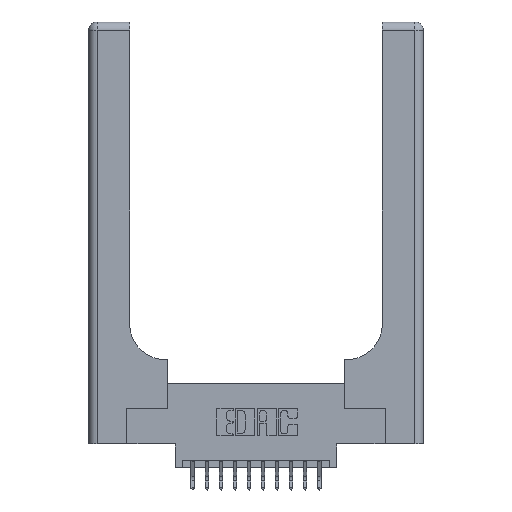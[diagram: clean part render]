
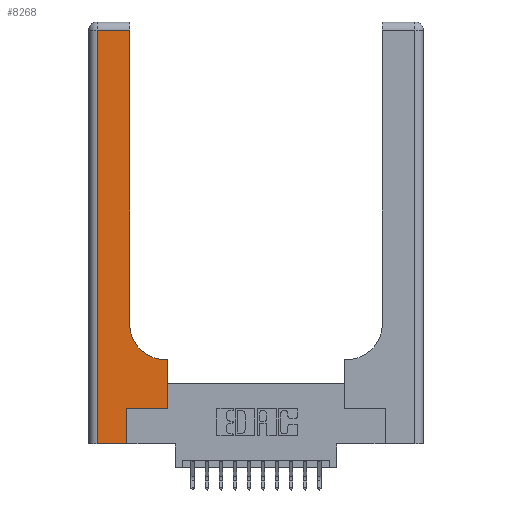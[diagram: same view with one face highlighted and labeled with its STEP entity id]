
A CAD part, top view. The second image highlights one B-rep face of the part: STEP entity #8268.
In plain terms, the highlighted planar face has unit normal (0, 0, 1).
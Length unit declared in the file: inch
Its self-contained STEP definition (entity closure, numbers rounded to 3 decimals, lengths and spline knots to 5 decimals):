
#43 = EDGE_CURVE ( 'NONE', #12131, #6065, #13467, .T. ) ;
#388 = CARTESIAN_POINT ( 'NONE',  ( 0.2915, 0.6, 0.37 ) ) ;
#536 = VECTOR ( 'NONE', #3226, 39.37008 ) ;
#683 = EDGE_CURVE ( 'NONE', #10627, #5318, #9512, .T. ) ;
#843 = CARTESIAN_POINT ( 'NONE',  ( 0., 0., 0.37 ) ) ;
#898 = ORIENTED_EDGE ( 'NONE', *, *, #2068, .T. ) ;
#954 = AXIS2_PLACEMENT_3D ( 'NONE', #13021, #5045, #14367 ) ;
#1008 = LINE ( 'NONE', #12621, #536 ) ;
#1689 = CARTESIAN_POINT ( 'NONE',  ( 0.06, 2.94, 0.37 ) ) ;
#2019 = CARTESIAN_POINT ( 'NONE',  ( 0.269, 0.25, 0.37 ) ) ;
#2068 = EDGE_CURVE ( 'NONE', #7461, #10627, #8013, .T. ) ;
#2261 = VECTOR ( 'NONE', #15564, 39.37008 ) ;
#3097 = DIRECTION ( 'NONE',  ( -1., 0., 0. ) ) ;
#3226 = DIRECTION ( 'NONE',  ( 0., 1., 0. ) ) ;
#3343 = DIRECTION ( 'NONE',  ( 0., -1., 0. ) ) ;
#4192 = EDGE_CURVE ( 'NONE', #5415, #10243, #4500, .T. ) ;
#4274 = ORIENTED_EDGE ( 'NONE', *, *, #10267, .T. ) ;
#4484 = CARTESIAN_POINT ( 'NONE',  ( 0., 2.94, 0.37 ) ) ;
#4500 = LINE ( 'NONE', #4484, #4947 ) ;
#4870 = DIRECTION ( 'NONE',  ( 1., 0., 0. ) ) ;
#4947 = VECTOR ( 'NONE', #3097, 39.37008 ) ;
#5045 = DIRECTION ( 'NONE',  ( 0., 0., -1. ) ) ;
#5318 = VERTEX_POINT ( 'NONE', #13586 ) ;
#5415 = VERTEX_POINT ( 'NONE', #11178 ) ;
#6065 = VERTEX_POINT ( 'NONE', #7530 ) ;
#6084 = CARTESIAN_POINT ( 'NONE',  ( 0.06, 3., 0.37 ) ) ;
#6275 = VECTOR ( 'NONE', #12805, 39.37008 ) ;
#6757 = CARTESIAN_POINT ( 'NONE',  ( 0.5415, 0.85, 0.37 ) ) ;
#6781 = CARTESIAN_POINT ( 'NONE',  ( 0.5585, 0.25, 0.37 ) ) ;
#6958 = LINE ( 'NONE', #388, #17168 ) ;
#7461 = VERTEX_POINT ( 'NONE', #11286 ) ;
#7468 = DIRECTION ( 'NONE',  ( -1., 0., 0. ) ) ;
#7530 = CARTESIAN_POINT ( 'NONE',  ( 0.269, 0., 0.37 ) ) ;
#7727 = VECTOR ( 'NONE', #3343, 39.37008 ) ;
#7764 = CIRCLE ( 'NONE', #10862, 0.25 ) ;
#7832 = EDGE_CURVE ( 'NONE', #16924, #9497, #7764, .T. ) ;
#8013 = LINE ( 'NONE', #2019, #11161 ) ;
#8097 = DIRECTION ( 'NONE',  ( 1., 0., 0. ) ) ;
#8153 = EDGE_CURVE ( 'NONE', #9497, #5415, #13346, .T. ) ;
#8268 = ADVANCED_FACE ( 'NONE', ( #14812 ), #9021, .F. ) ;
#8719 = ORIENTED_EDGE ( 'NONE', *, *, #16309, .T. ) ;
#8729 = EDGE_CURVE ( 'NONE', #10243, #12131, #11706, .T. ) ;
#8798 = CARTESIAN_POINT ( 'NONE',  ( 0.2915, 3., 0.37 ) ) ;
#9021 = PLANE ( 'NONE',  #954 ) ;
#9127 = ORIENTED_EDGE ( 'NONE', *, *, #7832, .T. ) ;
#9267 = EDGE_LOOP ( 'NONE', ( #10160, #17262, #10572, #14534, #4274, #898, #11847, #8719, #9127 ) ) ;
#9497 = VERTEX_POINT ( 'NONE', #12981 ) ;
#9512 = LINE ( 'NONE', #15324, #2261 ) ;
#9939 = VECTOR ( 'NONE', #17641, 39.37008 ) ;
#10058 = CARTESIAN_POINT ( 'NONE',  ( 0.06, 0., 0.37 ) ) ;
#10160 = ORIENTED_EDGE ( 'NONE', *, *, #8153, .T. ) ;
#10243 = VERTEX_POINT ( 'NONE', #1689 ) ;
#10267 = EDGE_CURVE ( 'NONE', #6065, #7461, #1008, .T. ) ;
#10572 = ORIENTED_EDGE ( 'NONE', *, *, #8729, .T. ) ;
#10627 = VERTEX_POINT ( 'NONE', #6781 ) ;
#10862 = AXIS2_PLACEMENT_3D ( 'NONE', #6757, #16089, #8097 ) ;
#11161 = VECTOR ( 'NONE', #4870, 39.37008 ) ;
#11178 = CARTESIAN_POINT ( 'NONE',  ( 0.2915, 2.94, 0.37 ) ) ;
#11286 = CARTESIAN_POINT ( 'NONE',  ( 0.269, 0.25, 0.37 ) ) ;
#11706 = LINE ( 'NONE', #6084, #7727 ) ;
#11847 = ORIENTED_EDGE ( 'NONE', *, *, #683, .T. ) ;
#12131 = VERTEX_POINT ( 'NONE', #10058 ) ;
#12621 = CARTESIAN_POINT ( 'NONE',  ( 0.269, 0., 0.37 ) ) ;
#12730 = CARTESIAN_POINT ( 'NONE',  ( 0.5415, 0.6, 0.37 ) ) ;
#12805 = DIRECTION ( 'NONE',  ( 0., 1., 0. ) ) ;
#12981 = CARTESIAN_POINT ( 'NONE',  ( 0.2915, 0.85, 0.37 ) ) ;
#13021 = CARTESIAN_POINT ( 'NONE',  ( 0., 3., 0.37 ) ) ;
#13346 = LINE ( 'NONE', #8798, #6275 ) ;
#13467 = LINE ( 'NONE', #843, #9939 ) ;
#13586 = CARTESIAN_POINT ( 'NONE',  ( 0.5585, 0.6, 0.37 ) ) ;
#14367 = DIRECTION ( 'NONE',  ( -1., 0., 0. ) ) ;
#14534 = ORIENTED_EDGE ( 'NONE', *, *, #43, .T. ) ;
#14812 = FACE_OUTER_BOUND ( 'NONE', #9267, .T. ) ;
#15324 = CARTESIAN_POINT ( 'NONE',  ( 0.5585, 0.25, 0.37 ) ) ;
#15564 = DIRECTION ( 'NONE',  ( 0., 1., 0. ) ) ;
#16089 = DIRECTION ( 'NONE',  ( 0., 0., -1. ) ) ;
#16309 = EDGE_CURVE ( 'NONE', #5318, #16924, #6958, .T. ) ;
#16924 = VERTEX_POINT ( 'NONE', #12730 ) ;
#17168 = VECTOR ( 'NONE', #7468, 39.37008 ) ;
#17262 = ORIENTED_EDGE ( 'NONE', *, *, #4192, .T. ) ;
#17641 = DIRECTION ( 'NONE',  ( 1., 0., 0. ) ) ;
